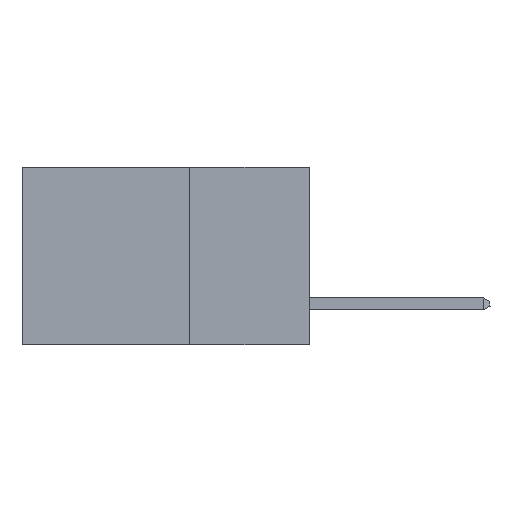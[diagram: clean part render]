
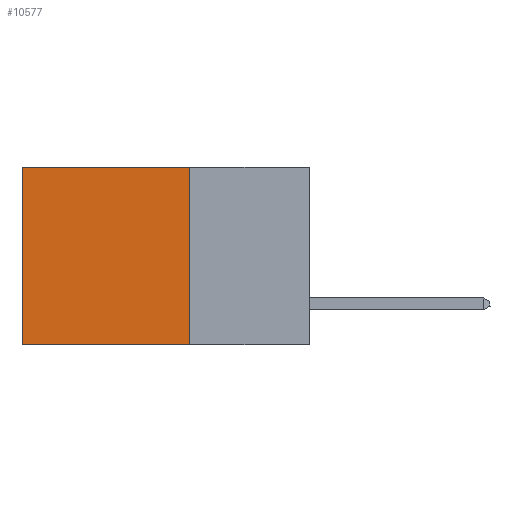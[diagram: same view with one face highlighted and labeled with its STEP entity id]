
A CAD part, left-side view. The second image highlights one B-rep face of the part: STEP entity #10577.
In plain terms, the highlighted planar face has unit normal (-1, 0, 0).
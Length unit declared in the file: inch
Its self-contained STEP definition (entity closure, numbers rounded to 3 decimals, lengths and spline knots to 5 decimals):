
#1363 = ORIENTED_EDGE ( 'NONE', *, *, #30920, .T. ) ;
#3349 = EDGE_CURVE ( 'NONE', #10199, #19652, #22902, .T. ) ;
#4673 = ORIENTED_EDGE ( 'NONE', *, *, #20391, .F. ) ;
#4781 = VECTOR ( 'NONE', #26326, 39.37008 ) ;
#4882 = EDGE_LOOP ( 'NONE', ( #1363, #4673, #26167, #18377 ) ) ;
#5023 = CARTESIAN_POINT ( 'NONE',  ( 0.2875, 0.25, 0. ) ) ;
#6075 = VERTEX_POINT ( 'NONE', #20359 ) ;
#6360 = VECTOR ( 'NONE', #11135, 39.37008 ) ;
#7198 = CARTESIAN_POINT ( 'NONE',  ( 0.2875, 0.25, 0. ) ) ;
#7331 = AXIS2_PLACEMENT_3D ( 'NONE', #5023, #29504, #24624 ) ;
#8253 = VERTEX_POINT ( 'NONE', #23695 ) ;
#9973 = VECTOR ( 'NONE', #12026, 39.37008 ) ;
#10199 = VERTEX_POINT ( 'NONE', #17740 ) ;
#10577 = ADVANCED_FACE ( 'NONE', ( #11042 ), #21517, .F. ) ;
#11013 = DIRECTION ( 'NONE',  ( 0., 1., 0. ) ) ;
#11042 = FACE_OUTER_BOUND ( 'NONE', #4882, .T. ) ;
#11135 = DIRECTION ( 'NONE',  ( 0., 0., -1. ) ) ;
#12026 = DIRECTION ( 'NONE',  ( 0., 1., 0. ) ) ;
#13518 = CARTESIAN_POINT ( 'NONE',  ( 0.2875, 0.6, 0. ) ) ;
#17740 = CARTESIAN_POINT ( 'NONE',  ( 0.2875, 0.25, 0. ) ) ;
#18232 = LINE ( 'NONE', #7198, #4781 ) ;
#18377 = ORIENTED_EDGE ( 'NONE', *, *, #3349, .T. ) ;
#18848 = CARTESIAN_POINT ( 'NONE',  ( 0.2875, 0.6, 0. ) ) ;
#19652 = VERTEX_POINT ( 'NONE', #18848 ) ;
#20359 = CARTESIAN_POINT ( 'NONE',  ( 0.2875, 0.25, -0.37 ) ) ;
#20391 = EDGE_CURVE ( 'NONE', #6075, #8253, #26764, .T. ) ;
#21517 = PLANE ( 'NONE',  #7331 ) ;
#22902 = LINE ( 'NONE', #25599, #24348 ) ;
#23695 = CARTESIAN_POINT ( 'NONE',  ( 0.2875, 0.6, -0.37 ) ) ;
#24348 = VECTOR ( 'NONE', #11013, 39.37008 ) ;
#24624 = DIRECTION ( 'NONE',  ( 0., 0., -1. ) ) ;
#25599 = CARTESIAN_POINT ( 'NONE',  ( 0.2875, 0.25, 0. ) ) ;
#26167 = ORIENTED_EDGE ( 'NONE', *, *, #29074, .F. ) ;
#26324 = CARTESIAN_POINT ( 'NONE',  ( 0.2875, 0.25, -0.37 ) ) ;
#26326 = DIRECTION ( 'NONE',  ( 0., 0., -1. ) ) ;
#26764 = LINE ( 'NONE', #26324, #9973 ) ;
#28060 = LINE ( 'NONE', #13518, #6360 ) ;
#29074 = EDGE_CURVE ( 'NONE', #10199, #6075, #18232, .T. ) ;
#29504 = DIRECTION ( 'NONE',  ( 1., 0., 0. ) ) ;
#30920 = EDGE_CURVE ( 'NONE', #19652, #8253, #28060, .T. ) ;
